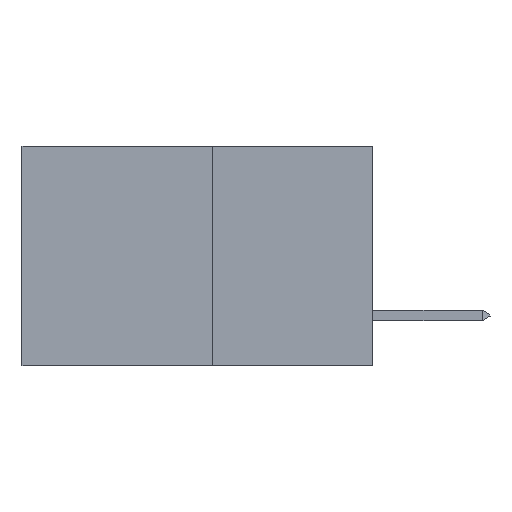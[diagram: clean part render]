
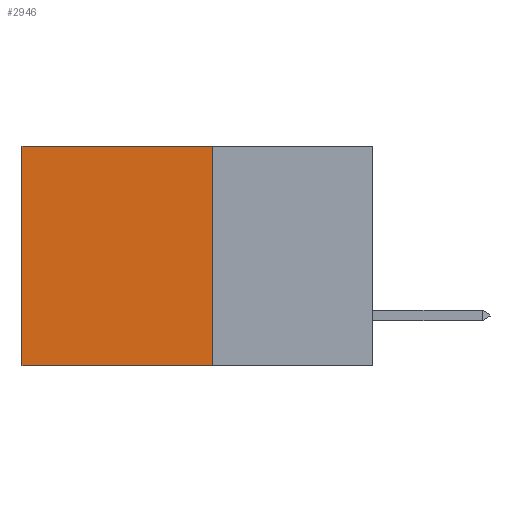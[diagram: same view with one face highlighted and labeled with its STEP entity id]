
A CAD part, left-side view. The second image highlights one B-rep face of the part: STEP entity #2946.
In plain terms, the highlighted planar face has unit normal (-1, 0, 0).
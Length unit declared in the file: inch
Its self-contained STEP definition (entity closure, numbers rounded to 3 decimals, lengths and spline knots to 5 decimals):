
#258 = CARTESIAN_POINT ( 'NONE',  ( 0.277, 0.59, -0.37 ) ) ;
#520 = VERTEX_POINT ( 'NONE', #2001 ) ;
#693 = LINE ( 'NONE', #14287, #7645 ) ;
#1658 = CARTESIAN_POINT ( 'NONE',  ( 0.277, 0.27, -0.37 ) ) ;
#2001 = CARTESIAN_POINT ( 'NONE',  ( 0.277, 0.27, -0.37 ) ) ;
#2195 = VECTOR ( 'NONE', #4247, 39.37008 ) ;
#2946 = ADVANCED_FACE ( 'NONE', ( #16272 ), #3733, .F. ) ;
#3151 = DIRECTION ( 'NONE',  ( 0., 0., -1. ) ) ;
#3561 = EDGE_CURVE ( 'NONE', #16610, #8354, #6633, .T. ) ;
#3733 = PLANE ( 'NONE',  #13676 ) ;
#3755 = CARTESIAN_POINT ( 'NONE',  ( 0.277, 0.27, -0.37 ) ) ;
#4247 = DIRECTION ( 'NONE',  ( 0., 1., 0. ) ) ;
#5221 = DIRECTION ( 'NONE',  ( 0., 0., -1. ) ) ;
#5287 = ORIENTED_EDGE ( 'NONE', *, *, #5530, .F. ) ;
#5530 = EDGE_CURVE ( 'NONE', #16610, #520, #14686, .T. ) ;
#5720 = DIRECTION ( 'NONE',  ( 0., 0., -1. ) ) ;
#6633 = LINE ( 'NONE', #10408, #2195 ) ;
#7367 = DIRECTION ( 'NONE',  ( 1., 0., 0. ) ) ;
#7645 = VECTOR ( 'NONE', #18398, 39.37008 ) ;
#8354 = VERTEX_POINT ( 'NONE', #18350 ) ;
#9474 = CARTESIAN_POINT ( 'NONE',  ( 0.277, 0.59, -0.37 ) ) ;
#10408 = CARTESIAN_POINT ( 'NONE',  ( 0.277, 0.27, 0. ) ) ;
#10628 = EDGE_LOOP ( 'NONE', ( #12391, #16072, #5287, #12819 ) ) ;
#12143 = EDGE_CURVE ( 'NONE', #8354, #13718, #14171, .T. ) ;
#12391 = ORIENTED_EDGE ( 'NONE', *, *, #12143, .T. ) ;
#12540 = CARTESIAN_POINT ( 'NONE',  ( 0.277, 0.27, 0. ) ) ;
#12819 = ORIENTED_EDGE ( 'NONE', *, *, #3561, .T. ) ;
#13676 = AXIS2_PLACEMENT_3D ( 'NONE', #3755, #7367, #5720 ) ;
#13718 = VERTEX_POINT ( 'NONE', #258 ) ;
#13737 = VECTOR ( 'NONE', #5221, 39.37008 ) ;
#14171 = LINE ( 'NONE', #9474, #13737 ) ;
#14248 = VECTOR ( 'NONE', #3151, 39.37008 ) ;
#14287 = CARTESIAN_POINT ( 'NONE',  ( 0.277, 0.27, -0.37 ) ) ;
#14686 = LINE ( 'NONE', #1658, #14248 ) ;
#16072 = ORIENTED_EDGE ( 'NONE', *, *, #18133, .F. ) ;
#16272 = FACE_OUTER_BOUND ( 'NONE', #10628, .T. ) ;
#16610 = VERTEX_POINT ( 'NONE', #12540 ) ;
#18133 = EDGE_CURVE ( 'NONE', #520, #13718, #693, .T. ) ;
#18350 = CARTESIAN_POINT ( 'NONE',  ( 0.277, 0.59, 0. ) ) ;
#18398 = DIRECTION ( 'NONE',  ( 0., 1., 0. ) ) ;
